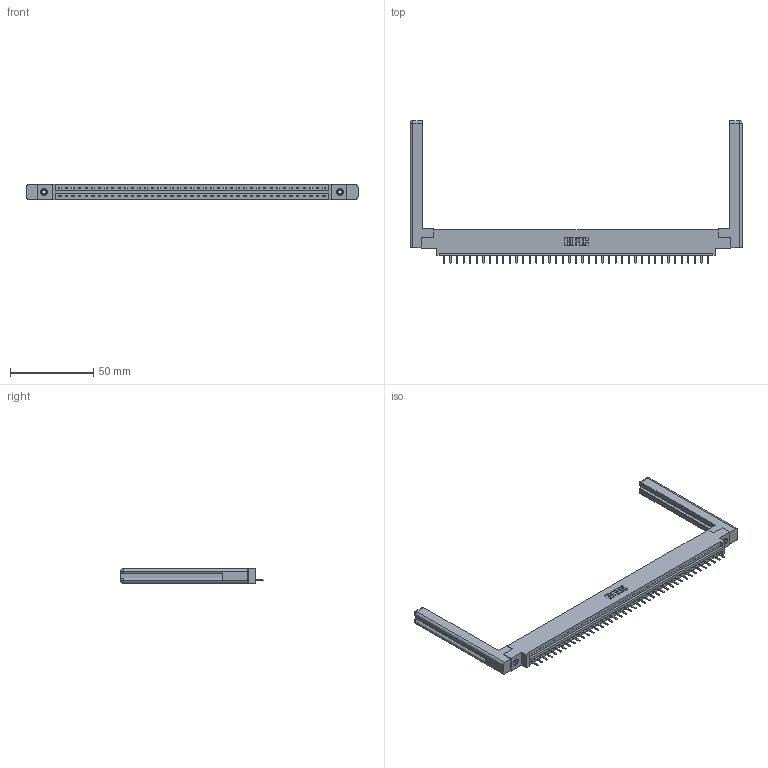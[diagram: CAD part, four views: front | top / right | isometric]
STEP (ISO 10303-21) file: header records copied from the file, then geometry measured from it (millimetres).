
FILE_DESCRIPTION (( 'STEP AP203' ), '1' );
FILE_NAME ('337-041-520-658.STEP', '2019-10-01T20:26:32', ( '' ), ( '' ), 'SwSTEP 2.0', 'SolidWorks 2016', '' );
FILE_SCHEMA (( 'CONFIG_CONTROL_DESIGN' ));
Length unit declared in the file: inch
Products named in the file (5): 345-250-001_345-250-001-102; 345-292-001_345-293-120; 337-041-520-658; 337 Part_0.170 Offset - 0.156 Dia-TI; 307-220-058
Assembly tree (46 placements, depth 2):
  337-041-520-658
    337 Part_0.170 Offset - 0.156 Dia-TI
    345-292-001_345-293-120  x41
    345-250-001_345-250-001-102  x2
    307-220-058  x2
Bounding box: 199.09 x 85.43 x 9.4 mm (x, y, z)
Volume: 27605.8 mm3; surface area: 26004.8 mm2
Topology: 46 solids, 46 shells, 2966 faces, 8713 edges, 5686 vertices
Faces by surface type: plane 2126, cylinder 816, cone 12, torus 12
Entity records: 33486 total; most frequent: CARTESIAN_POINT 5844, ORIENTED_EDGE 5748, DIRECTION 4928, EDGE_CURVE 2874, VECTOR 2694, LINE 2694, VERTEX_POINT 1906, AXIS2_PLACEMENT_3D 1117
